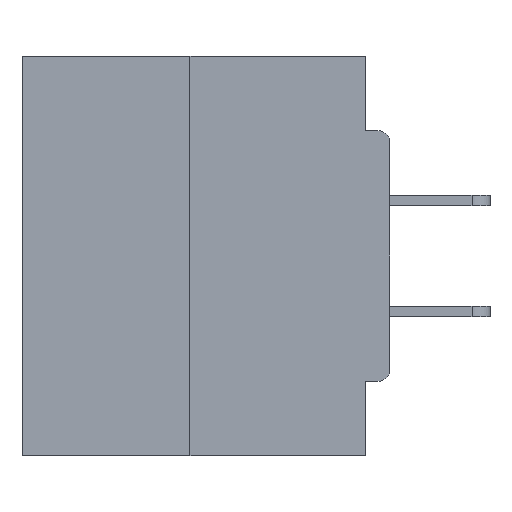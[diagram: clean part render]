
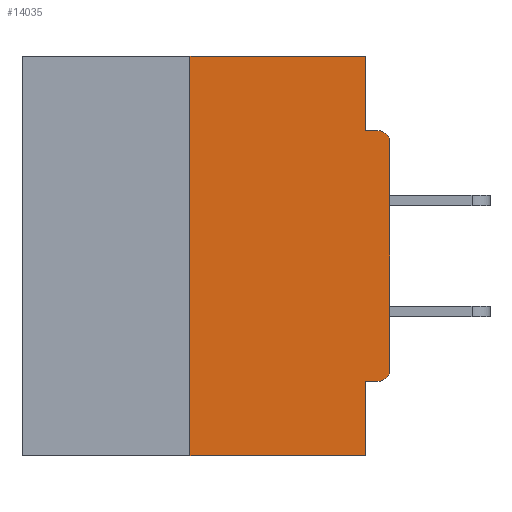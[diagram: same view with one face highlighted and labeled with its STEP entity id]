
A CAD part, left-side view. The second image highlights one B-rep face of the part: STEP entity #14035.
In plain terms, the highlighted planar face has unit normal (-1, 0, 0).
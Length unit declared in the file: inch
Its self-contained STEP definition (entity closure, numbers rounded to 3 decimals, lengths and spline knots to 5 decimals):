
#171 = ORIENTED_EDGE ( 'NONE', *, *, #23552, .T. ) ;
#297 = VERTEX_POINT ( 'NONE', #28735 ) ;
#605 = CARTESIAN_POINT ( 'NONE',  ( 0., 0.25, -0.5 ) ) ;
#1173 = VECTOR ( 'NONE', #12696, 39.37008 ) ;
#1323 = ORIENTED_EDGE ( 'NONE', *, *, #19888, .F. ) ;
#1417 = EDGE_CURVE ( 'NONE', #30899, #297, #16697, .T. ) ;
#1666 = CARTESIAN_POINT ( 'NONE',  ( 0., 0.015, -0.1085 ) ) ;
#2318 = EDGE_CURVE ( 'NONE', #11362, #25346, #19484, .T. ) ;
#2760 = DIRECTION ( 'NONE',  ( 0., -1., 0. ) ) ;
#3160 = CARTESIAN_POINT ( 'NONE',  ( 0., 0.46, 0. ) ) ;
#3205 = LINE ( 'NONE', #20732, #10738 ) ;
#3654 = CARTESIAN_POINT ( 'NONE',  ( 0., 0.46, 0. ) ) ;
#3724 = LINE ( 'NONE', #11159, #30114 ) ;
#4407 = VERTEX_POINT ( 'NONE', #5876 ) ;
#4535 = EDGE_CURVE ( 'NONE', #9942, #31150, #3724, .T. ) ;
#5061 = VECTOR ( 'NONE', #15644, 39.37008 ) ;
#5361 = VERTEX_POINT ( 'NONE', #27644 ) ;
#5578 = LINE ( 'NONE', #28150, #1173 ) ;
#5876 = CARTESIAN_POINT ( 'NONE',  ( 0., 0.015, -0.4065 ) ) ;
#6198 = CARTESIAN_POINT ( 'NONE',  ( 0., 0., -0.1085 ) ) ;
#6238 = ORIENTED_EDGE ( 'NONE', *, *, #33096, .F. ) ;
#7266 = CIRCLE ( 'NONE', #12844, 0.015 ) ;
#7530 = AXIS2_PLACEMENT_3D ( 'NONE', #3654, #28913, #13551 ) ;
#8580 = DIRECTION ( 'NONE',  ( 0., 0., -1. ) ) ;
#9329 = DIRECTION ( 'NONE',  ( 0., 0., -1. ) ) ;
#9846 = VECTOR ( 'NONE', #12804, 39.37008 ) ;
#9942 = VERTEX_POINT ( 'NONE', #10017 ) ;
#10017 = CARTESIAN_POINT ( 'NONE',  ( 0., 0.031, -0.0935 ) ) ;
#10738 = VECTOR ( 'NONE', #26094, 39.37008 ) ;
#11075 = ORIENTED_EDGE ( 'NONE', *, *, #2318, .F. ) ;
#11159 = CARTESIAN_POINT ( 'NONE',  ( 0., 0., -0.0935 ) ) ;
#11362 = VERTEX_POINT ( 'NONE', #605 ) ;
#11786 = DIRECTION ( 'NONE',  ( -1., 0., 0. ) ) ;
#11811 = CARTESIAN_POINT ( 'NONE',  ( 0., 0.031, -0.4065 ) ) ;
#11916 = DIRECTION ( 'NONE',  ( -1., 0., 0. ) ) ;
#12033 = EDGE_LOOP ( 'NONE', ( #23370, #11075, #171, #20912, #1323, #28298, #26519, #13654, #26941, #6238 ) ) ;
#12060 = VECTOR ( 'NONE', #2760, 39.37008 ) ;
#12092 = LINE ( 'NONE', #12983, #12060 ) ;
#12473 = CARTESIAN_POINT ( 'NONE',  ( 0., 0.015, -0.0935 ) ) ;
#12696 = DIRECTION ( 'NONE',  ( 0., 1., 0. ) ) ;
#12804 = DIRECTION ( 'NONE',  ( 0., 0., 1. ) ) ;
#12844 = AXIS2_PLACEMENT_3D ( 'NONE', #19238, #11916, #19464 ) ;
#12983 = CARTESIAN_POINT ( 'NONE',  ( 0., 0.46, -0.5 ) ) ;
#13156 = CARTESIAN_POINT ( 'NONE',  ( 0., 0.25, 0. ) ) ;
#13551 = DIRECTION ( 'NONE',  ( 0., 0., -1. ) ) ;
#13654 = ORIENTED_EDGE ( 'NONE', *, *, #23259, .T. ) ;
#14035 = ADVANCED_FACE ( 'NONE', ( #15168 ), #24230, .F. ) ;
#15168 = FACE_OUTER_BOUND ( 'NONE', #12033, .T. ) ;
#15644 = DIRECTION ( 'NONE',  ( 0., -1., 0. ) ) ;
#16317 = CARTESIAN_POINT ( 'NONE',  ( 0., 0.031, 0. ) ) ;
#16697 = LINE ( 'NONE', #19229, #22700 ) ;
#17018 = VERTEX_POINT ( 'NONE', #6198 ) ;
#17042 = LINE ( 'NONE', #3160, #5061 ) ;
#18747 = CARTESIAN_POINT ( 'NONE',  ( 0., 0.25, 0. ) ) ;
#19229 = CARTESIAN_POINT ( 'NONE',  ( 0., 0.031, -0.5 ) ) ;
#19238 = CARTESIAN_POINT ( 'NONE',  ( 0., 0.015, -0.3915 ) ) ;
#19464 = DIRECTION ( 'NONE',  ( 0., 0., -1. ) ) ;
#19484 = LINE ( 'NONE', #13156, #9846 ) ;
#19580 = EDGE_CURVE ( 'NONE', #24069, #17018, #3205, .T. ) ;
#19888 = EDGE_CURVE ( 'NONE', #4407, #30899, #5578, .T. ) ;
#20732 = CARTESIAN_POINT ( 'NONE',  ( 0., 0., 0. ) ) ;
#20912 = ORIENTED_EDGE ( 'NONE', *, *, #1417, .F. ) ;
#21009 = AXIS2_PLACEMENT_3D ( 'NONE', #1666, #11786, #9329 ) ;
#21571 = EDGE_CURVE ( 'NONE', #25346, #5361, #17042, .T. ) ;
#22700 = VECTOR ( 'NONE', #26575, 39.37008 ) ;
#23259 = EDGE_CURVE ( 'NONE', #17018, #31150, #31322, .T. ) ;
#23370 = ORIENTED_EDGE ( 'NONE', *, *, #21571, .F. ) ;
#23552 = EDGE_CURVE ( 'NONE', #11362, #297, #12092, .T. ) ;
#24069 = VERTEX_POINT ( 'NONE', #31271 ) ;
#24230 = PLANE ( 'NONE',  #7530 ) ;
#24387 = LINE ( 'NONE', #16317, #25567 ) ;
#24750 = EDGE_CURVE ( 'NONE', #4407, #24069, #7266, .T. ) ;
#25346 = VERTEX_POINT ( 'NONE', #18747 ) ;
#25567 = VECTOR ( 'NONE', #8580, 39.37008 ) ;
#26094 = DIRECTION ( 'NONE',  ( 0., 0., 1. ) ) ;
#26519 = ORIENTED_EDGE ( 'NONE', *, *, #19580, .T. ) ;
#26575 = DIRECTION ( 'NONE',  ( 0., 0., -1. ) ) ;
#26941 = ORIENTED_EDGE ( 'NONE', *, *, #4535, .F. ) ;
#27644 = CARTESIAN_POINT ( 'NONE',  ( 0., 0.031, 0. ) ) ;
#28150 = CARTESIAN_POINT ( 'NONE',  ( 0., 0., -0.4065 ) ) ;
#28298 = ORIENTED_EDGE ( 'NONE', *, *, #24750, .T. ) ;
#28735 = CARTESIAN_POINT ( 'NONE',  ( 0., 0.031, -0.5 ) ) ;
#28913 = DIRECTION ( 'NONE',  ( 1., 0., 0. ) ) ;
#29210 = DIRECTION ( 'NONE',  ( 0., -1., 0. ) ) ;
#30114 = VECTOR ( 'NONE', #29210, 39.37008 ) ;
#30899 = VERTEX_POINT ( 'NONE', #11811 ) ;
#31150 = VERTEX_POINT ( 'NONE', #12473 ) ;
#31271 = CARTESIAN_POINT ( 'NONE',  ( 0., 0., -0.3915 ) ) ;
#31322 = CIRCLE ( 'NONE', #21009, 0.015 ) ;
#33096 = EDGE_CURVE ( 'NONE', #5361, #9942, #24387, .T. ) ;
